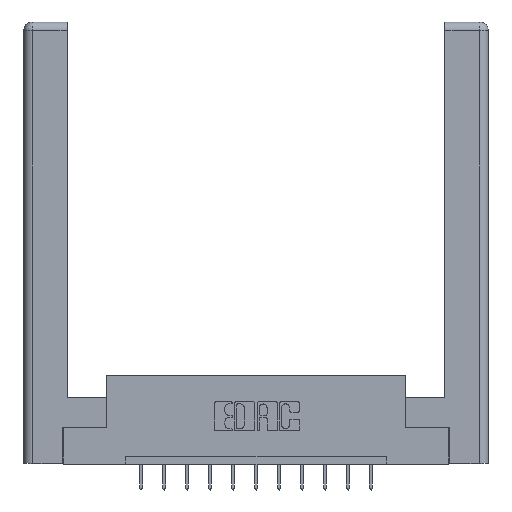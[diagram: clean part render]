
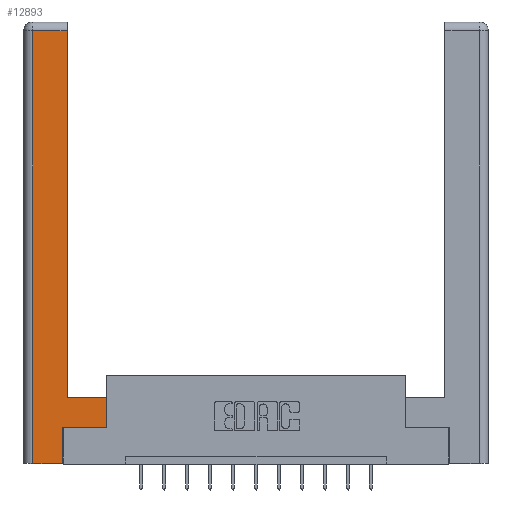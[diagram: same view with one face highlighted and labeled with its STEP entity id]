
A CAD part, top view. The second image highlights one B-rep face of the part: STEP entity #12893.
In plain terms, the highlighted planar face has unit normal (0, 0, 1).
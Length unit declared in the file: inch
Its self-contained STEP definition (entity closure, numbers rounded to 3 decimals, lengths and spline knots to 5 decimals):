
#3 = CARTESIAN_POINT ( 'NONE',  ( 0.0615, 2.94, 0. ) ) ;
#311 = VERTEX_POINT ( 'NONE', #11071 ) ;
#340 = VERTEX_POINT ( 'NONE', #13544 ) ;
#532 = ORIENTED_EDGE ( 'NONE', *, *, #3363, .T. ) ;
#600 = CARTESIAN_POINT ( 'NONE',  ( 0.0615, 0., 0. ) ) ;
#816 = ORIENTED_EDGE ( 'NONE', *, *, #8353, .T. ) ;
#1297 = VERTEX_POINT ( 'NONE', #14576 ) ;
#1615 = ORIENTED_EDGE ( 'NONE', *, *, #8794, .T. ) ;
#2022 = EDGE_CURVE ( 'NONE', #340, #7156, #7823, .T. ) ;
#2301 = VECTOR ( 'NONE', #3476, 39.37008 ) ;
#2846 = CARTESIAN_POINT ( 'NONE',  ( 0.0615, 0., 0. ) ) ;
#3196 = DIRECTION ( 'NONE',  ( 1., 0., 0. ) ) ;
#3363 = EDGE_CURVE ( 'NONE', #7579, #4944, #7809, .T. ) ;
#3476 = DIRECTION ( 'NONE',  ( -1., 0., 0. ) ) ;
#4099 = LINE ( 'NONE', #7854, #4279 ) ;
#4279 = VECTOR ( 'NONE', #12406, 39.37008 ) ;
#4387 = DIRECTION ( 'NONE',  ( 0., 1., 0. ) ) ;
#4724 = CARTESIAN_POINT ( 'NONE',  ( 0.295, 0.45, 0. ) ) ;
#4944 = VERTEX_POINT ( 'NONE', #10100 ) ;
#5025 = VECTOR ( 'NONE', #10337, 39.37008 ) ;
#5214 = EDGE_LOOP ( 'NONE', ( #14586, #816, #5610, #532, #13708, #7957, #9529, #1615 ) ) ;
#5439 = VECTOR ( 'NONE', #3196, 39.37008 ) ;
#5464 = CARTESIAN_POINT ( 'NONE',  ( 0., 0., 0. ) ) ;
#5610 = ORIENTED_EDGE ( 'NONE', *, *, #13434, .T. ) ;
#5765 = AXIS2_PLACEMENT_3D ( 'NONE', #5464, #10155, #11365 ) ;
#5907 = CARTESIAN_POINT ( 'NONE',  ( 0.295, 3., 0. ) ) ;
#5973 = EDGE_CURVE ( 'NONE', #4944, #12370, #7629, .T. ) ;
#6732 = VECTOR ( 'NONE', #13855, 39.37008 ) ;
#7051 = EDGE_CURVE ( 'NONE', #311, #1297, #7782, .T. ) ;
#7156 = VERTEX_POINT ( 'NONE', #12223 ) ;
#7272 = VECTOR ( 'NONE', #7933, 39.37008 ) ;
#7579 = VERTEX_POINT ( 'NONE', #2846 ) ;
#7629 = LINE ( 'NONE', #11278, #11586 ) ;
#7782 = LINE ( 'NONE', #11282, #13549 ) ;
#7809 = LINE ( 'NONE', #13454, #5439 ) ;
#7823 = LINE ( 'NONE', #5907, #6732 ) ;
#7854 = CARTESIAN_POINT ( 'NONE',  ( 0.565, 0.245, 0. ) ) ;
#7933 = DIRECTION ( 'NONE',  ( 0., -1., 0. ) ) ;
#7957 = ORIENTED_EDGE ( 'NONE', *, *, #10941, .T. ) ;
#8353 = EDGE_CURVE ( 'NONE', #7156, #11386, #11514, .T. ) ;
#8794 = EDGE_CURVE ( 'NONE', #1297, #340, #9142, .T. ) ;
#8995 = PLANE ( 'NONE',  #5765 ) ;
#9142 = LINE ( 'NONE', #4724, #2301 ) ;
#9529 = ORIENTED_EDGE ( 'NONE', *, *, #7051, .T. ) ;
#9911 = DIRECTION ( 'NONE',  ( 0., 1., 0. ) ) ;
#10100 = CARTESIAN_POINT ( 'NONE',  ( 0.265, 0., 0. ) ) ;
#10155 = DIRECTION ( 'NONE',  ( 0., 0., -1. ) ) ;
#10337 = DIRECTION ( 'NONE',  ( -1., 0., 0. ) ) ;
#10351 = LINE ( 'NONE', #600, #7272 ) ;
#10364 = FACE_OUTER_BOUND ( 'NONE', #5214, .T. ) ;
#10941 = EDGE_CURVE ( 'NONE', #12370, #311, #4099, .T. ) ;
#11071 = CARTESIAN_POINT ( 'NONE',  ( 0.565, 0.245, 0. ) ) ;
#11278 = CARTESIAN_POINT ( 'NONE',  ( 0.265, 0.245, 0. ) ) ;
#11282 = CARTESIAN_POINT ( 'NONE',  ( 0.565, 0.45, 0. ) ) ;
#11365 = DIRECTION ( 'NONE',  ( -1., 0., 0. ) ) ;
#11386 = VERTEX_POINT ( 'NONE', #3 ) ;
#11496 = CARTESIAN_POINT ( 'NONE',  ( 0.0615, 2.94, 0. ) ) ;
#11514 = LINE ( 'NONE', #11496, #5025 ) ;
#11586 = VECTOR ( 'NONE', #9911, 39.37008 ) ;
#12005 = CARTESIAN_POINT ( 'NONE',  ( 0.265, 0.245, 0. ) ) ;
#12223 = CARTESIAN_POINT ( 'NONE',  ( 0.295, 2.94, 0. ) ) ;
#12370 = VERTEX_POINT ( 'NONE', #12005 ) ;
#12406 = DIRECTION ( 'NONE',  ( 1., 0., 0. ) ) ;
#12893 = ADVANCED_FACE ( 'NONE', ( #10364 ), #8995, .F. ) ;
#13434 = EDGE_CURVE ( 'NONE', #11386, #7579, #10351, .T. ) ;
#13454 = CARTESIAN_POINT ( 'NONE',  ( 0.265, 0., 0. ) ) ;
#13544 = CARTESIAN_POINT ( 'NONE',  ( 0.295, 0.45, 0. ) ) ;
#13549 = VECTOR ( 'NONE', #4387, 39.37008 ) ;
#13708 = ORIENTED_EDGE ( 'NONE', *, *, #5973, .T. ) ;
#13855 = DIRECTION ( 'NONE',  ( 0., 1., 0. ) ) ;
#14576 = CARTESIAN_POINT ( 'NONE',  ( 0.565, 0.45, 0. ) ) ;
#14586 = ORIENTED_EDGE ( 'NONE', *, *, #2022, .T. ) ;
